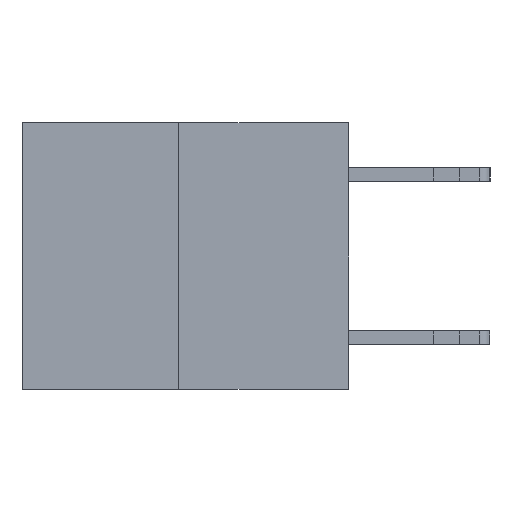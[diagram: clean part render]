
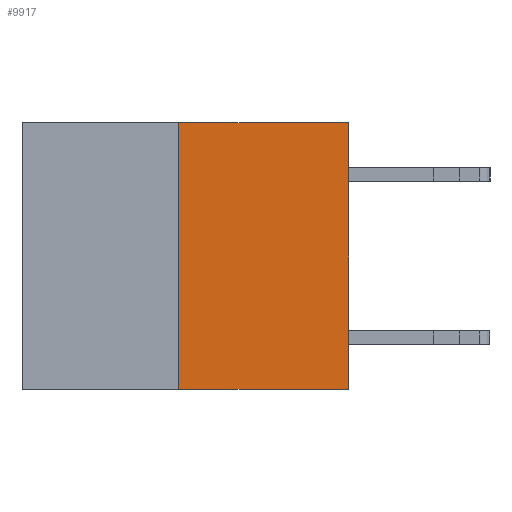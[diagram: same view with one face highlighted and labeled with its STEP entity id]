
A CAD part, left-side view. The second image highlights one B-rep face of the part: STEP entity #9917.
In plain terms, the highlighted planar face has unit normal (-1, 0, 0).
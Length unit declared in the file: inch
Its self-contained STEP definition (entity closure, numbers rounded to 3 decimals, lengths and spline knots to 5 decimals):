
#30 = VERTEX_POINT ( 'NONE', #4148 ) ;
#406 = DIRECTION ( 'NONE',  ( 0., 0., 1. ) ) ;
#530 = AXIS2_PLACEMENT_3D ( 'NONE', #9170, #3735, #10327 ) ;
#557 = DIRECTION ( 'NONE',  ( 0., -1., 0. ) ) ;
#709 = PLANE ( 'NONE',  #530 ) ;
#1007 = CARTESIAN_POINT ( 'NONE',  ( 0., 0., -0.49 ) ) ;
#1019 = ORIENTED_EDGE ( 'NONE', *, *, #13451, .F. ) ;
#1683 = CARTESIAN_POINT ( 'NONE',  ( 0., 0.6, -0.49 ) ) ;
#1901 = EDGE_CURVE ( 'NONE', #12149, #30, #2230, .T. ) ;
#2230 = LINE ( 'NONE', #2626, #13396 ) ;
#2316 = VERTEX_POINT ( 'NONE', #11894 ) ;
#2626 = CARTESIAN_POINT ( 'NONE',  ( 0., 0., 0. ) ) ;
#3156 = VECTOR ( 'NONE', #557, 39.37008 ) ;
#3735 = DIRECTION ( 'NONE',  ( 1., 0., 0. ) ) ;
#3821 = CARTESIAN_POINT ( 'NONE',  ( 0., 0.6, 0. ) ) ;
#4117 = VECTOR ( 'NONE', #12118, 39.37008 ) ;
#4148 = CARTESIAN_POINT ( 'NONE',  ( 0., 0., 0. ) ) ;
#4199 = DIRECTION ( 'NONE',  ( 0., -1., 0. ) ) ;
#4759 = LINE ( 'NONE', #6301, #4117 ) ;
#6301 = CARTESIAN_POINT ( 'NONE',  ( 0., 0.312, -0.49 ) ) ;
#6442 = VERTEX_POINT ( 'NONE', #8298 ) ;
#6638 = ORIENTED_EDGE ( 'NONE', *, *, #9539, .T. ) ;
#6819 = ORIENTED_EDGE ( 'NONE', *, *, #1901, .T. ) ;
#7428 = VECTOR ( 'NONE', #4199, 39.37008 ) ;
#8114 = LINE ( 'NONE', #3821, #7428 ) ;
#8298 = CARTESIAN_POINT ( 'NONE',  ( 0., 0.312, 0. ) ) ;
#8626 = LINE ( 'NONE', #1683, #3156 ) ;
#9013 = EDGE_LOOP ( 'NONE', ( #1019, #6638, #6819, #10186 ) ) ;
#9170 = CARTESIAN_POINT ( 'NONE',  ( 0., 0.6, 0. ) ) ;
#9539 = EDGE_CURVE ( 'NONE', #2316, #12149, #8626, .T. ) ;
#9917 = ADVANCED_FACE ( 'NONE', ( #10160 ), #709, .F. ) ;
#10160 = FACE_OUTER_BOUND ( 'NONE', #9013, .T. ) ;
#10186 = ORIENTED_EDGE ( 'NONE', *, *, #10199, .F. ) ;
#10199 = EDGE_CURVE ( 'NONE', #6442, #30, #8114, .T. ) ;
#10327 = DIRECTION ( 'NONE',  ( 0., 0., -1. ) ) ;
#11894 = CARTESIAN_POINT ( 'NONE',  ( 0., 0.312, -0.49 ) ) ;
#12118 = DIRECTION ( 'NONE',  ( 0., 0., 1. ) ) ;
#12149 = VERTEX_POINT ( 'NONE', #1007 ) ;
#13396 = VECTOR ( 'NONE', #406, 39.37008 ) ;
#13451 = EDGE_CURVE ( 'NONE', #2316, #6442, #4759, .T. ) ;
